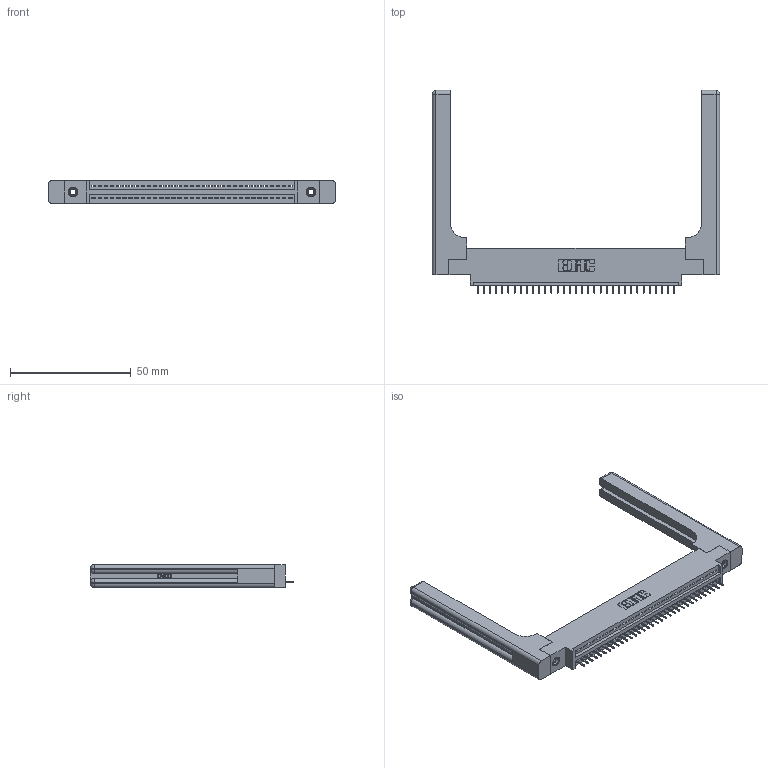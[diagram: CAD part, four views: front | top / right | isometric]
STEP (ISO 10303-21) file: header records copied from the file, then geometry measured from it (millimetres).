
FILE_DESCRIPTION (( 'STEP AP203' ), '1' );
FILE_NAME ('395-033-525-658.STEP', '2020-09-23T21:57:31', ( '' ), ( '' ), 'SwSTEP 2.0', 'SolidWorks 2020', '' );
FILE_SCHEMA (( 'CONFIG_CONTROL_DESIGN' ));
Length unit declared in the file: inch
Products named in the file (5): 395-033-525-658; 345 Part_0.170 Offset - 0.156 Dia-TH; 345-292-001_345-293-125; 345-220-058_345-220-058; 345-250-001_345-250-001-102
Assembly tree (38 placements, depth 2):
  395-033-525-658
    345 Part_0.170 Offset - 0.156 Dia-TH
    345-292-001_345-293-125  x33
    345-250-001_345-250-001-102  x2
    345-220-058_345-220-058  x2
Bounding box: 118.85 x 84 x 9.4 mm (x, y, z)
Volume: 19471.3 mm3; surface area: 19433.7 mm2
Topology: 38 solids, 38 shells, 2432 faces, 6959 edges, 4486 vertices
Faces by surface type: plane 1750, cylinder 622, bspline 36, cone 12, sphere 8, torus 4
Entity records: 31436 total; most frequent: CARTESIAN_POINT 6416, ORIENTED_EDGE 5180, DIRECTION 4564, EDGE_CURVE 2590, LINE 2238, VECTOR 2238, VERTEX_POINT 1714, AXIS2_PLACEMENT_3D 1163
